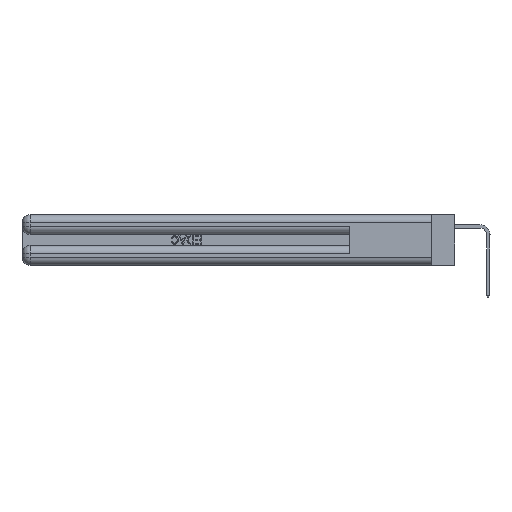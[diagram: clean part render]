
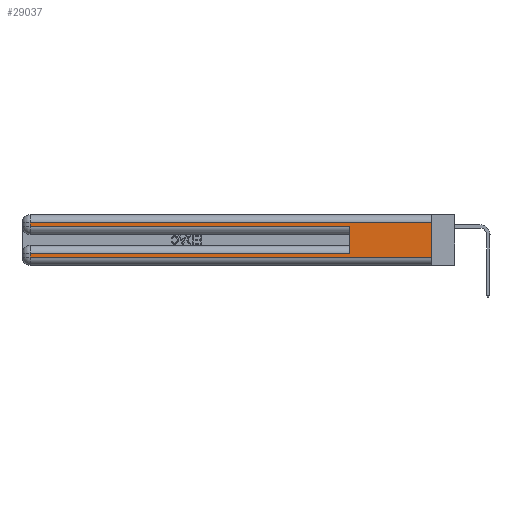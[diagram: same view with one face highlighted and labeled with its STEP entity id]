
A CAD part, left-side view. The second image highlights one B-rep face of the part: STEP entity #29037.
In plain terms, the highlighted planar face has unit normal (-1, 0, 0).
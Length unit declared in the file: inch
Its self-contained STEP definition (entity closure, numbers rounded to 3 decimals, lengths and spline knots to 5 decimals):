
#106 = ORIENTED_EDGE ( 'NONE', *, *, #36642, .T. ) ;
#1016 = LINE ( 'NONE', #26555, #35214 ) ;
#1143 = EDGE_LOOP ( 'NONE', ( #36858, #106, #3799, #7766, #20914, #3489, #20122, #23650 ) ) ;
#2130 = DIRECTION ( 'NONE',  ( 1., 0., 0. ) ) ;
#2786 = CARTESIAN_POINT ( 'NONE',  ( 0., 2.94, 0.06 ) ) ;
#3489 = ORIENTED_EDGE ( 'NONE', *, *, #8788, .T. ) ;
#3591 = VERTEX_POINT ( 'NONE', #33767 ) ;
#3658 = VECTOR ( 'NONE', #28245, 39.37008 ) ;
#3799 = ORIENTED_EDGE ( 'NONE', *, *, #28167, .T. ) ;
#4846 = VECTOR ( 'NONE', #24523, 39.37008 ) ;
#7128 = DIRECTION ( 'NONE',  ( 0., 1., 0. ) ) ;
#7766 = ORIENTED_EDGE ( 'NONE', *, *, #26001, .T. ) ;
#8231 = AXIS2_PLACEMENT_3D ( 'NONE', #21476, #2130, #24682 ) ;
#8514 = LINE ( 'NONE', #11575, #32088 ) ;
#8788 = EDGE_CURVE ( 'NONE', #23975, #17395, #30883, .T. ) ;
#10198 = CARTESIAN_POINT ( 'NONE',  ( 0., 2.94, 0.37 ) ) ;
#10551 = DIRECTION ( 'NONE',  ( 0., -1., 0. ) ) ;
#11575 = CARTESIAN_POINT ( 'NONE',  ( 0., 0., 0.06 ) ) ;
#11720 = DIRECTION ( 'NONE',  ( 0., 0., -1. ) ) ;
#12097 = CARTESIAN_POINT ( 'NONE',  ( 0., 2.94, 0.085 ) ) ;
#14877 = DIRECTION ( 'NONE',  ( 0., 0., -1. ) ) ;
#14903 = VERTEX_POINT ( 'NONE', #39057 ) ;
#14933 = CARTESIAN_POINT ( 'NONE',  ( 0., 2.94, 0.37 ) ) ;
#17395 = VERTEX_POINT ( 'NONE', #12097 ) ;
#17410 = EDGE_CURVE ( 'NONE', #23975, #3591, #38664, .T. ) ;
#17980 = CARTESIAN_POINT ( 'NONE',  ( 0., 0., 0.37 ) ) ;
#18882 = CARTESIAN_POINT ( 'NONE',  ( 0., 2.94, 0.285 ) ) ;
#20122 = ORIENTED_EDGE ( 'NONE', *, *, #37404, .T. ) ;
#20567 = CARTESIAN_POINT ( 'NONE',  ( 0., 0., 0.06 ) ) ;
#20628 = VECTOR ( 'NONE', #23124, 39.37008 ) ;
#20914 = ORIENTED_EDGE ( 'NONE', *, *, #17410, .F. ) ;
#21429 = LINE ( 'NONE', #14933, #37316 ) ;
#21476 = CARTESIAN_POINT ( 'NONE',  ( 0., 0., 0.37 ) ) ;
#23124 = DIRECTION ( 'NONE',  ( 0., 0., -1. ) ) ;
#23609 = VERTEX_POINT ( 'NONE', #23652 ) ;
#23650 = ORIENTED_EDGE ( 'NONE', *, *, #35327, .T. ) ;
#23652 = CARTESIAN_POINT ( 'NONE',  ( 0., 2.94, 0.31 ) ) ;
#23975 = VERTEX_POINT ( 'NONE', #25292 ) ;
#24467 = DIRECTION ( 'NONE',  ( 0., -1., 0. ) ) ;
#24523 = DIRECTION ( 'NONE',  ( 0., 1., 0. ) ) ;
#24682 = DIRECTION ( 'NONE',  ( 0., 0., -1. ) ) ;
#25001 = CARTESIAN_POINT ( 'NONE',  ( 0., 0.6, 0.145 ) ) ;
#25292 = CARTESIAN_POINT ( 'NONE',  ( 0., 0.6, 0.085 ) ) ;
#26001 = EDGE_CURVE ( 'NONE', #29813, #3591, #1016, .T. ) ;
#26317 = VECTOR ( 'NONE', #14877, 39.37008 ) ;
#26555 = CARTESIAN_POINT ( 'NONE',  ( 0., 0., 0.285 ) ) ;
#27336 = LINE ( 'NONE', #17980, #26317 ) ;
#28068 = FACE_OUTER_BOUND ( 'NONE', #1143, .T. ) ;
#28167 = EDGE_CURVE ( 'NONE', #23609, #29813, #29152, .T. ) ;
#28245 = DIRECTION ( 'NONE',  ( 0., 0., 1. ) ) ;
#29037 = ADVANCED_FACE ( 'NONE', ( #28068 ), #40428, .F. ) ;
#29152 = LINE ( 'NONE', #10198, #20628 ) ;
#29589 = CARTESIAN_POINT ( 'NONE',  ( 0., 0., 0.085 ) ) ;
#29813 = VERTEX_POINT ( 'NONE', #18882 ) ;
#30500 = LINE ( 'NONE', #37141, #4846 ) ;
#30883 = LINE ( 'NONE', #29589, #37262 ) ;
#31661 = VERTEX_POINT ( 'NONE', #2786 ) ;
#32088 = VECTOR ( 'NONE', #24467, 39.37008 ) ;
#33142 = VERTEX_POINT ( 'NONE', #20567 ) ;
#33767 = CARTESIAN_POINT ( 'NONE',  ( 0., 0.6, 0.285 ) ) ;
#35214 = VECTOR ( 'NONE', #10551, 39.37008 ) ;
#35327 = EDGE_CURVE ( 'NONE', #31661, #33142, #8514, .T. ) ;
#36642 = EDGE_CURVE ( 'NONE', #14903, #23609, #30500, .T. ) ;
#36858 = ORIENTED_EDGE ( 'NONE', *, *, #38699, .F. ) ;
#37141 = CARTESIAN_POINT ( 'NONE',  ( 0., 0., 0.31 ) ) ;
#37262 = VECTOR ( 'NONE', #7128, 39.37008 ) ;
#37316 = VECTOR ( 'NONE', #11720, 39.37008 ) ;
#37404 = EDGE_CURVE ( 'NONE', #17395, #31661, #21429, .T. ) ;
#38664 = LINE ( 'NONE', #25001, #3658 ) ;
#38699 = EDGE_CURVE ( 'NONE', #14903, #33142, #27336, .T. ) ;
#39057 = CARTESIAN_POINT ( 'NONE',  ( 0., 0., 0.31 ) ) ;
#40428 = PLANE ( 'NONE',  #8231 ) ;
